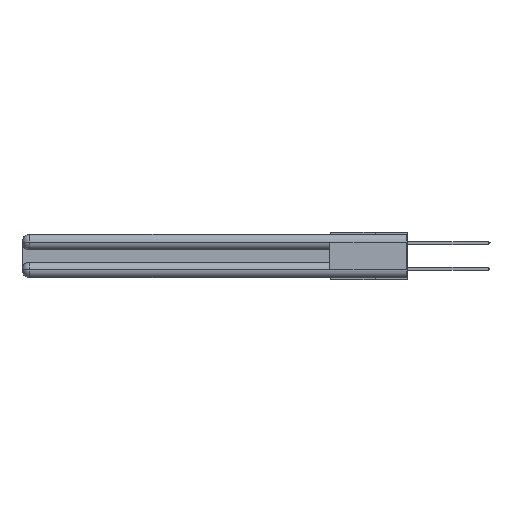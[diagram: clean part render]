
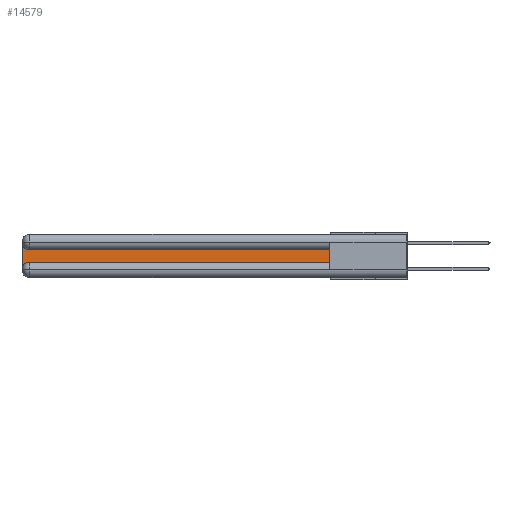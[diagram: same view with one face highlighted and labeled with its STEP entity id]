
A CAD part, left-side view. The second image highlights one B-rep face of the part: STEP entity #14579.
In plain terms, the highlighted planar face has unit normal (-1, 0, 0).
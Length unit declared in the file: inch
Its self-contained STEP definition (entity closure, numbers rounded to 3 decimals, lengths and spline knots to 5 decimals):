
#761 = ORIENTED_EDGE ( 'NONE', *, *, #30517, .T. ) ;
#1111 = CARTESIAN_POINT ( 'NONE',  ( 0.075, 0.6, -0.2175 ) ) ;
#1490 = PLANE ( 'NONE',  #15492 ) ;
#1790 = AXIS2_PLACEMENT_3D ( 'NONE', #27154, #32746, #29834 ) ;
#2216 = CARTESIAN_POINT ( 'NONE',  ( 0.075, 0.6, -0.1225 ) ) ;
#2436 = DIRECTION ( 'NONE',  ( 0., 1., 0. ) ) ;
#3259 = VERTEX_POINT ( 'NONE', #12704 ) ;
#3550 = EDGE_CURVE ( 'NONE', #6755, #3259, #15366, .T. ) ;
#3640 = VERTEX_POINT ( 'NONE', #1111 ) ;
#3800 = VECTOR ( 'NONE', #14112, 39.37008 ) ;
#4555 = DIRECTION ( 'NONE',  ( 0., 0., -1. ) ) ;
#5580 = ORIENTED_EDGE ( 'NONE', *, *, #31166, .T. ) ;
#5973 = LINE ( 'NONE', #9862, #13973 ) ;
#6419 = DIRECTION ( 'NONE',  ( 1., 0., 0. ) ) ;
#6652 = DIRECTION ( 'NONE',  ( 0., 0., -1. ) ) ;
#6755 = VERTEX_POINT ( 'NONE', #26596 ) ;
#7841 = VECTOR ( 'NONE', #2436, 39.37008 ) ;
#8205 = ORIENTED_EDGE ( 'NONE', *, *, #26510, .T. ) ;
#8267 = CARTESIAN_POINT ( 'NONE',  ( 0.075, 2.94, -0.2775 ) ) ;
#9862 = CARTESIAN_POINT ( 'NONE',  ( 0.075, 3., -0.2175 ) ) ;
#10277 = EDGE_CURVE ( 'NONE', #18510, #6755, #24522, .T. ) ;
#11370 = CARTESIAN_POINT ( 'NONE',  ( 0.075, 0.6, -0.2175 ) ) ;
#12188 = VECTOR ( 'NONE', #30481, 39.37008 ) ;
#12212 = ORIENTED_EDGE ( 'NONE', *, *, #13835, .T. ) ;
#12704 = CARTESIAN_POINT ( 'NONE',  ( 0.075, 3., -0.0625 ) ) ;
#13835 = EDGE_CURVE ( 'NONE', #23812, #25778, #31156, .T. ) ;
#13973 = VECTOR ( 'NONE', #4555, 39.37008 ) ;
#14112 = DIRECTION ( 'NONE',  ( 0., 0., 1. ) ) ;
#14579 = ADVANCED_FACE ( 'NONE', ( #26103 ), #1490, .F. ) ;
#14715 = LINE ( 'NONE', #11370, #12188 ) ;
#15366 = CIRCLE ( 'NONE', #1790, 0.06 ) ;
#15492 = AXIS2_PLACEMENT_3D ( 'NONE', #22405, #6419, #6652 ) ;
#16132 = CARTESIAN_POINT ( 'NONE',  ( 0.075, 2.94, -0.2175 ) ) ;
#17694 = EDGE_LOOP ( 'NONE', ( #24237, #30959, #761, #12212, #8205, #5580 ) ) ;
#18510 = VERTEX_POINT ( 'NONE', #2216 ) ;
#19970 = AXIS2_PLACEMENT_3D ( 'NONE', #8267, #29485, #29124 ) ;
#22405 = CARTESIAN_POINT ( 'NONE',  ( 0.075, 3., -0.1225 ) ) ;
#23812 = VERTEX_POINT ( 'NONE', #26749 ) ;
#24237 = ORIENTED_EDGE ( 'NONE', *, *, #10277, .T. ) ;
#24522 = LINE ( 'NONE', #29051, #7841 ) ;
#25778 = VERTEX_POINT ( 'NONE', #16132 ) ;
#26103 = FACE_OUTER_BOUND ( 'NONE', #17694, .T. ) ;
#26510 = EDGE_CURVE ( 'NONE', #25778, #3640, #14715, .T. ) ;
#26596 = CARTESIAN_POINT ( 'NONE',  ( 0.075, 2.94, -0.1225 ) ) ;
#26749 = CARTESIAN_POINT ( 'NONE',  ( 0.075, 3., -0.2775 ) ) ;
#27016 = CARTESIAN_POINT ( 'NONE',  ( 0.075, 0.6, -0.2175 ) ) ;
#27154 = CARTESIAN_POINT ( 'NONE',  ( 0.075, 2.94, -0.0625 ) ) ;
#29051 = CARTESIAN_POINT ( 'NONE',  ( 0.075, 0.6, -0.1225 ) ) ;
#29124 = DIRECTION ( 'NONE',  ( 0., 0., -1. ) ) ;
#29485 = DIRECTION ( 'NONE',  ( 1., 0., 0. ) ) ;
#29834 = DIRECTION ( 'NONE',  ( 0., 0., -1. ) ) ;
#30481 = DIRECTION ( 'NONE',  ( 0., -1., 0. ) ) ;
#30517 = EDGE_CURVE ( 'NONE', #3259, #23812, #5973, .T. ) ;
#30562 = LINE ( 'NONE', #27016, #3800 ) ;
#30959 = ORIENTED_EDGE ( 'NONE', *, *, #3550, .T. ) ;
#31156 = CIRCLE ( 'NONE', #19970, 0.06 ) ;
#31166 = EDGE_CURVE ( 'NONE', #3640, #18510, #30562, .T. ) ;
#32746 = DIRECTION ( 'NONE',  ( 1., 0., 0. ) ) ;
